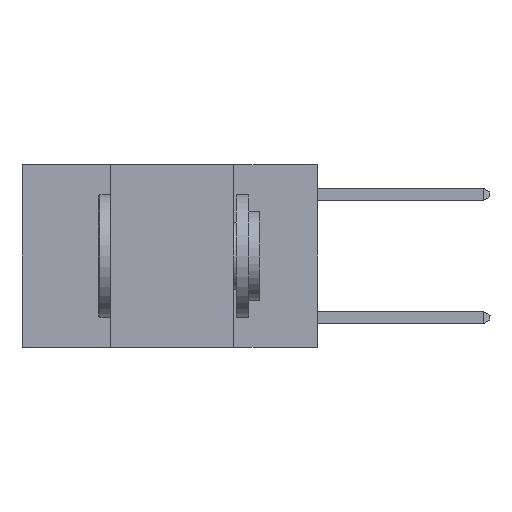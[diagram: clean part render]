
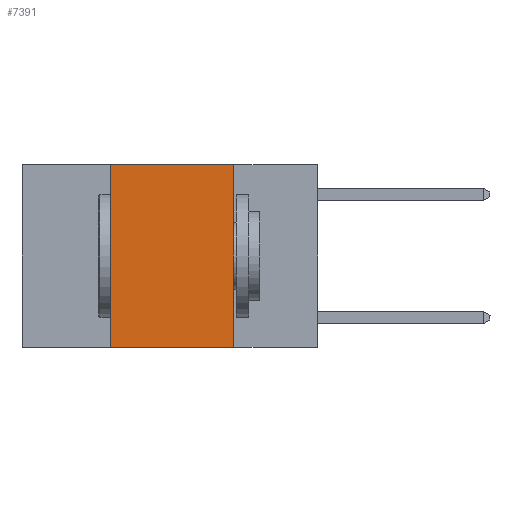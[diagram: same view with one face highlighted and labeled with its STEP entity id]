
A CAD part, left-side view. The second image highlights one B-rep face of the part: STEP entity #7391.
In plain terms, the highlighted planar face has unit normal (-1, 0, 0).
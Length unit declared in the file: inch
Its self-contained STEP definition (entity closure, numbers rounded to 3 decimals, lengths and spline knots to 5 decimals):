
#648 = CARTESIAN_POINT ( 'NONE',  ( 0., 0.42, 0. ) ) ;
#1291 = VECTOR ( 'NONE', #3209, 39.37008 ) ;
#1382 = DIRECTION ( 'NONE',  ( 0., 0., -1. ) ) ;
#1448 = VECTOR ( 'NONE', #6837, 39.37008 ) ;
#1712 = CARTESIAN_POINT ( 'NONE',  ( 0., 0.42, 0. ) ) ;
#1836 = VERTEX_POINT ( 'NONE', #648 ) ;
#1899 = LINE ( 'NONE', #6659, #8337 ) ;
#1901 = CARTESIAN_POINT ( 'NONE',  ( 0., 0.17, -0.37 ) ) ;
#2028 = VECTOR ( 'NONE', #7133, 39.37008 ) ;
#2409 = DIRECTION ( 'NONE',  ( 1., 0., 0. ) ) ;
#3209 = DIRECTION ( 'NONE',  ( 0., 0., 1. ) ) ;
#3251 = LINE ( 'NONE', #1712, #1291 ) ;
#3302 = EDGE_CURVE ( 'NONE', #8917, #5766, #4023, .T. ) ;
#3611 = ORIENTED_EDGE ( 'NONE', *, *, #3302, .T. ) ;
#3748 = AXIS2_PLACEMENT_3D ( 'NONE', #6944, #2409, #7653 ) ;
#4023 = LINE ( 'NONE', #4859, #2028 ) ;
#4532 = CARTESIAN_POINT ( 'NONE',  ( 0., 0.6, 0. ) ) ;
#4580 = CARTESIAN_POINT ( 'NONE',  ( 0., 0.17, 0. ) ) ;
#4788 = ORIENTED_EDGE ( 'NONE', *, *, #4839, .F. ) ;
#4799 = ORIENTED_EDGE ( 'NONE', *, *, #7470, .F. ) ;
#4824 = ORIENTED_EDGE ( 'NONE', *, *, #9123, .F. ) ;
#4839 = EDGE_CURVE ( 'NONE', #5679, #5766, #1899, .T. ) ;
#4859 = CARTESIAN_POINT ( 'NONE',  ( 0., 0.6, -0.37 ) ) ;
#5425 = PLANE ( 'NONE',  #3748 ) ;
#5679 = VERTEX_POINT ( 'NONE', #4580 ) ;
#5766 = VERTEX_POINT ( 'NONE', #1901 ) ;
#6659 = CARTESIAN_POINT ( 'NONE',  ( 0., 0.17, 0. ) ) ;
#6837 = DIRECTION ( 'NONE',  ( 0., -1., 0. ) ) ;
#6944 = CARTESIAN_POINT ( 'NONE',  ( 0., 0.6, 0. ) ) ;
#7133 = DIRECTION ( 'NONE',  ( 0., -1., 0. ) ) ;
#7329 = CARTESIAN_POINT ( 'NONE',  ( 0., 0.42, -0.37 ) ) ;
#7391 = ADVANCED_FACE ( 'NONE', ( #7719 ), #5425, .F. ) ;
#7470 = EDGE_CURVE ( 'NONE', #8917, #1836, #3251, .T. ) ;
#7653 = DIRECTION ( 'NONE',  ( 0., 0., -1. ) ) ;
#7719 = FACE_OUTER_BOUND ( 'NONE', #7897, .T. ) ;
#7897 = EDGE_LOOP ( 'NONE', ( #4788, #4824, #4799, #3611 ) ) ;
#8337 = VECTOR ( 'NONE', #1382, 39.37008 ) ;
#8917 = VERTEX_POINT ( 'NONE', #7329 ) ;
#9123 = EDGE_CURVE ( 'NONE', #1836, #5679, #9353, .T. ) ;
#9353 = LINE ( 'NONE', #4532, #1448 ) ;
